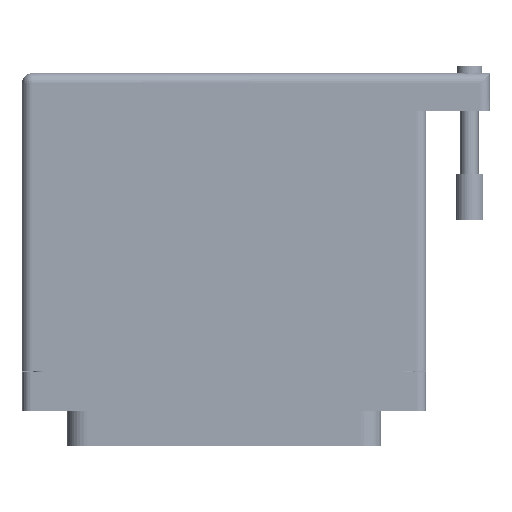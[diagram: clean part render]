
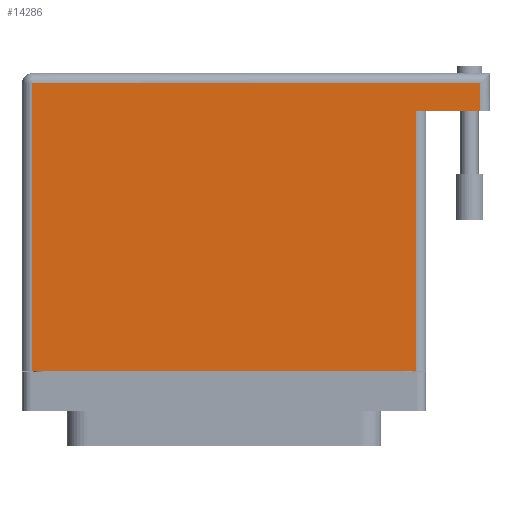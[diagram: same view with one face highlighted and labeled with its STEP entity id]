
A CAD part, front view. The second image highlights one B-rep face of the part: STEP entity #14286.
In plain terms, the highlighted face is planar.
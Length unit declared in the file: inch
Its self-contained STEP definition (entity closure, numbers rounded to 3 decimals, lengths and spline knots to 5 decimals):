
#875 = VERTEX_POINT ( 'NONE', #16255 ) ;
#1082 = EDGE_CURVE ( 'NONE', #37246, #87194, #13515, .T. ) ;
#2768 = EDGE_CURVE ( 'NONE', #87194, #71059, #19661, .T. ) ;
#5291 = VECTOR ( 'NONE', #26515, 39.37008 ) ;
#11690 = EDGE_CURVE ( 'NONE', #63129, #50767, #44498, .T. ) ;
#12795 = CARTESIAN_POINT ( 'NONE',  ( 1.3075, 1.674, 0.765 ) ) ;
#13011 = ORIENTED_EDGE ( 'NONE', *, *, #2768, .T. ) ;
#13515 = LINE ( 'NONE', #88456, #84561 ) ;
#13867 = CARTESIAN_POINT ( 'NONE',  ( -1.3075, 1.86, 0.765 ) ) ;
#14286 = ADVANCED_FACE ( 'NONE', ( #17385 ), #50708, .F. ) ;
#16185 = EDGE_LOOP ( 'NONE', ( #13011, #44639, #48474, #58682, #85325, #88504 ) ) ;
#16255 = CARTESIAN_POINT ( 'NONE',  ( 1.7425, 1.86, 0.765 ) ) ;
#17385 = FACE_OUTER_BOUND ( 'NONE', #16185, .T. ) ;
#19661 = LINE ( 'NONE', #25327, #35734 ) ;
#25327 = CARTESIAN_POINT ( 'NONE',  ( -1.3775, -0.1, 0.765 ) ) ;
#26515 = DIRECTION ( 'NONE',  ( 0., 1., 0. ) ) ;
#29104 = VECTOR ( 'NONE', #72713, 39.37008 ) ;
#32889 = CARTESIAN_POINT ( 'NONE',  ( 1.7425, 1.674, 0.765 ) ) ;
#34738 = DIRECTION ( 'NONE',  ( -1., 0., 0. ) ) ;
#35734 = VECTOR ( 'NONE', #45146, 39.37008 ) ;
#36539 = DIRECTION ( 'NONE',  ( 0., 0., -1. ) ) ;
#37246 = VERTEX_POINT ( 'NONE', #13867 ) ;
#40215 = DIRECTION ( 'NONE',  ( 0., -1., 0. ) ) ;
#44498 = LINE ( 'NONE', #48898, #82257 ) ;
#44639 = ORIENTED_EDGE ( 'NONE', *, *, #59359, .T. ) ;
#45146 = DIRECTION ( 'NONE',  ( 1., 0., 0. ) ) ;
#48474 = ORIENTED_EDGE ( 'NONE', *, *, #11690, .F. ) ;
#48898 = CARTESIAN_POINT ( 'NONE',  ( 1.8125, 1.674, 0.765 ) ) ;
#50708 = PLANE ( 'NONE',  #64483 ) ;
#50767 = VERTEX_POINT ( 'NONE', #12795 ) ;
#51884 = CARTESIAN_POINT ( 'NONE',  ( 1.3075, -0.1, 0.765 ) ) ;
#54343 = CARTESIAN_POINT ( 'NONE',  ( -1.3075, -0.1, 0.765 ) ) ;
#58682 = ORIENTED_EDGE ( 'NONE', *, *, #81779, .T. ) ;
#59359 = EDGE_CURVE ( 'NONE', #71059, #50767, #83989, .T. ) ;
#60757 = CARTESIAN_POINT ( 'NONE',  ( 1.7425, 1.93, 0.765 ) ) ;
#61481 = VECTOR ( 'NONE', #84800, 39.37008 ) ;
#63129 = VERTEX_POINT ( 'NONE', #32889 ) ;
#63772 = EDGE_CURVE ( 'NONE', #875, #37246, #87355, .T. ) ;
#64483 = AXIS2_PLACEMENT_3D ( 'NONE', #71792, #36539, #85358 ) ;
#65806 = CARTESIAN_POINT ( 'NONE',  ( 1.3075, 1.674, 0.765 ) ) ;
#71059 = VERTEX_POINT ( 'NONE', #51884 ) ;
#71792 = CARTESIAN_POINT ( 'NONE',  ( -1.3775, 1.93, 0.765 ) ) ;
#72713 = DIRECTION ( 'NONE',  ( 0., 1., 0. ) ) ;
#78448 = LINE ( 'NONE', #60757, #5291 ) ;
#81779 = EDGE_CURVE ( 'NONE', #63129, #875, #78448, .T. ) ;
#82257 = VECTOR ( 'NONE', #34738, 39.37008 ) ;
#83621 = CARTESIAN_POINT ( 'NONE',  ( -1.3775, 1.86, 0.765 ) ) ;
#83989 = LINE ( 'NONE', #65806, #29104 ) ;
#84561 = VECTOR ( 'NONE', #40215, 39.37008 ) ;
#84800 = DIRECTION ( 'NONE',  ( -1., 0., 0. ) ) ;
#85325 = ORIENTED_EDGE ( 'NONE', *, *, #63772, .T. ) ;
#85358 = DIRECTION ( 'NONE',  ( -1., 0., 0. ) ) ;
#87194 = VERTEX_POINT ( 'NONE', #54343 ) ;
#87355 = LINE ( 'NONE', #83621, #61481 ) ;
#88456 = CARTESIAN_POINT ( 'NONE',  ( -1.3075, -0.1, 0.765 ) ) ;
#88504 = ORIENTED_EDGE ( 'NONE', *, *, #1082, .T. ) ;
